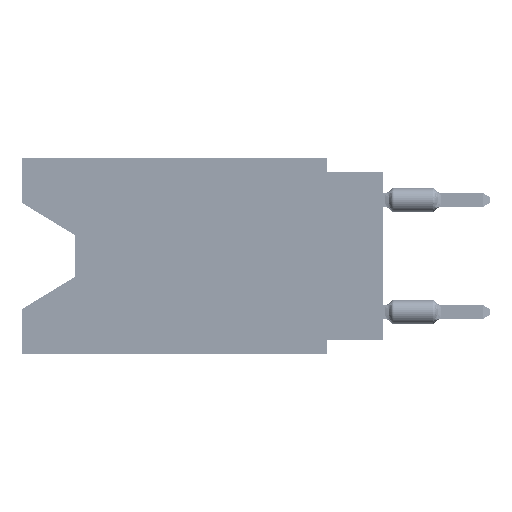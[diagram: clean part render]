
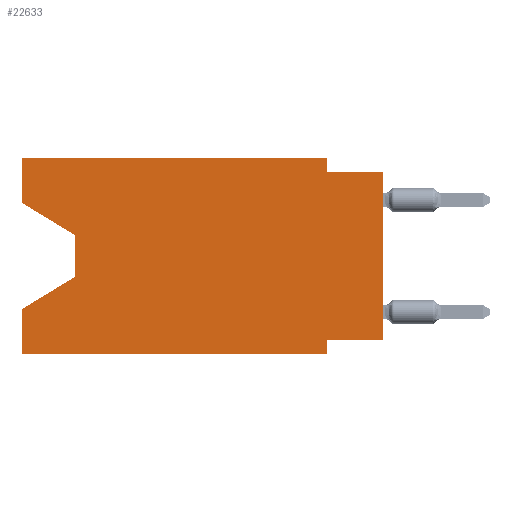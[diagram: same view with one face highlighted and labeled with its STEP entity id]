
A CAD part, left-side view. The second image highlights one B-rep face of the part: STEP entity #22633.
In plain terms, the highlighted planar face has unit normal (-1, 0, 0).
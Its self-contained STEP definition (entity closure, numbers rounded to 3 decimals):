
#1457 = LINE ( 'NONE', #22696, #9150 ) ;
#1768 = VERTEX_POINT ( 'NONE', #43482 ) ;
#1957 = VECTOR ( 'NONE', #57188, 1000. ) ;
#2181 = LINE ( 'NONE', #44290, #11183 ) ;
#2239 = DIRECTION ( 'NONE',  ( 0., 0., 1. ) ) ;
#2450 = EDGE_CURVE ( 'NONE', #53971, #31366, #9779, .T. ) ;
#2933 = EDGE_CURVE ( 'NONE', #52639, #45383, #1457, .T. ) ;
#3321 = DIRECTION ( 'NONE',  ( 0., 0., -1. ) ) ;
#3591 = LINE ( 'NONE', #34068, #43857 ) ;
#5191 = CARTESIAN_POINT ( 'NONE',  ( 0., 13.97, -3.505 ) ) ;
#8055 = CARTESIAN_POINT ( 'NONE',  ( 0., 16.383, 0. ) ) ;
#9150 = VECTOR ( 'NONE', #43224, 1000. ) ;
#9559 = VECTOR ( 'NONE', #39302, 1000. ) ;
#9779 = LINE ( 'NONE', #15256, #10186 ) ;
#10186 = VECTOR ( 'NONE', #26220, 1000. ) ;
#10486 = VERTEX_POINT ( 'NONE', #17986 ) ;
#10541 = FACE_OUTER_BOUND ( 'NONE', #41070, .T. ) ;
#11183 = VECTOR ( 'NONE', #33697, 1000. ) ;
#12348 = DIRECTION ( 'NONE',  ( 0., -1., 0. ) ) ;
#12874 = AXIS2_PLACEMENT_3D ( 'NONE', #35909, #58080, #63221 ) ;
#13448 = EDGE_CURVE ( 'NONE', #23213, #16446, #3591, .T. ) ;
#14159 = LINE ( 'NONE', #40508, #60738 ) ;
#15256 = CARTESIAN_POINT ( 'NONE',  ( 0., 0., -8.255 ) ) ;
#16075 = CARTESIAN_POINT ( 'NONE',  ( 0., 2.54, -8.255 ) ) ;
#16446 = VERTEX_POINT ( 'NONE', #31584 ) ;
#17041 = EDGE_CURVE ( 'NONE', #31366, #42974, #55352, .T. ) ;
#17986 = CARTESIAN_POINT ( 'NONE',  ( 0., 13.97, -3.505 ) ) ;
#18175 = CARTESIAN_POINT ( 'NONE',  ( 0., 16.383, -8.89 ) ) ;
#20119 = EDGE_CURVE ( 'NONE', #1768, #33820, #14159, .T. ) ;
#20193 = CARTESIAN_POINT ( 'NONE',  ( 0., 0., 0. ) ) ;
#20783 = CARTESIAN_POINT ( 'NONE',  ( 0., 2.54, -8.89 ) ) ;
#20844 = CARTESIAN_POINT ( 'NONE',  ( 0., 2.54, 0. ) ) ;
#20927 = VECTOR ( 'NONE', #12348, 1000. ) ;
#22633 = ADVANCED_FACE ( 'NONE', ( #10541 ), #31445, .F. ) ;
#22696 = CARTESIAN_POINT ( 'NONE',  ( 0., 16.383, 0. ) ) ;
#23194 = VECTOR ( 'NONE', #61239, 1000. ) ;
#23213 = VERTEX_POINT ( 'NONE', #60718 ) ;
#26065 = CARTESIAN_POINT ( 'NONE',  ( 0., 0., -0.635 ) ) ;
#26220 = DIRECTION ( 'NONE',  ( 0., 1., 0. ) ) ;
#26972 = CARTESIAN_POINT ( 'NONE',  ( 0., 16.383, 0. ) ) ;
#28565 = ORIENTED_EDGE ( 'NONE', *, *, #2450, .F. ) ;
#31091 = ORIENTED_EDGE ( 'NONE', *, *, #50137, .T. ) ;
#31366 = VERTEX_POINT ( 'NONE', #16075 ) ;
#31445 = PLANE ( 'NONE',  #12874 ) ;
#31584 = CARTESIAN_POINT ( 'NONE',  ( 0., 16.383, -6.852 ) ) ;
#31736 = CARTESIAN_POINT ( 'NONE',  ( 0., 2.54, 0. ) ) ;
#31999 = ORIENTED_EDGE ( 'NONE', *, *, #2933, .F. ) ;
#33697 = DIRECTION ( 'NONE',  ( 0., -0.855, -0.519 ) ) ;
#33820 = VERTEX_POINT ( 'NONE', #26065 ) ;
#33824 = CARTESIAN_POINT ( 'NONE',  ( 0., 2.54, -8.89 ) ) ;
#33839 = CARTESIAN_POINT ( 'NONE',  ( 0., 16.383, 0. ) ) ;
#34068 = CARTESIAN_POINT ( 'NONE',  ( 0., 13.97, -5.385 ) ) ;
#35244 = LINE ( 'NONE', #20844, #57721 ) ;
#35268 = ORIENTED_EDGE ( 'NONE', *, *, #37673, .F. ) ;
#35909 = CARTESIAN_POINT ( 'NONE',  ( 0., 16.383, 0. ) ) ;
#36280 = EDGE_CURVE ( 'NONE', #10486, #23213, #61992, .T. ) ;
#36671 = EDGE_CURVE ( 'NONE', #44117, #1768, #35244, .T. ) ;
#37070 = CARTESIAN_POINT ( 'NONE',  ( 0., 0., -8.255 ) ) ;
#37673 = EDGE_CURVE ( 'NONE', #45383, #44117, #63678, .T. ) ;
#39302 = DIRECTION ( 'NONE',  ( 0., -1., 0. ) ) ;
#40508 = CARTESIAN_POINT ( 'NONE',  ( 0., 0., -0.635 ) ) ;
#41070 = EDGE_LOOP ( 'NONE', ( #53090, #60513, #53792, #55802, #62577, #66275, #28565, #31091, #55437, #60100, #35268, #31999 ) ) ;
#42760 = VECTOR ( 'NONE', #2239, 1000. ) ;
#42974 = VERTEX_POINT ( 'NONE', #20783 ) ;
#43224 = DIRECTION ( 'NONE',  ( 0., 0., 1. ) ) ;
#43482 = CARTESIAN_POINT ( 'NONE',  ( 0., 2.54, -0.635 ) ) ;
#43857 = VECTOR ( 'NONE', #60406, 1000. ) ;
#44117 = VERTEX_POINT ( 'NONE', #31736 ) ;
#44290 = CARTESIAN_POINT ( 'NONE',  ( 0., 16.383, -2.038 ) ) ;
#44846 = LINE ( 'NONE', #20193, #23194 ) ;
#45383 = VERTEX_POINT ( 'NONE', #26972 ) ;
#49137 = LINE ( 'NONE', #8055, #42760 ) ;
#49919 = EDGE_CURVE ( 'NONE', #53029, #42974, #56932, .T. ) ;
#50137 = EDGE_CURVE ( 'NONE', #53971, #33820, #44846, .T. ) ;
#52412 = EDGE_CURVE ( 'NONE', #52639, #10486, #2181, .T. ) ;
#52639 = VERTEX_POINT ( 'NONE', #56217 ) ;
#53029 = VERTEX_POINT ( 'NONE', #62245 ) ;
#53090 = ORIENTED_EDGE ( 'NONE', *, *, #52412, .T. ) ;
#53792 = ORIENTED_EDGE ( 'NONE', *, *, #13448, .T. ) ;
#53971 = VERTEX_POINT ( 'NONE', #37070 ) ;
#55352 = LINE ( 'NONE', #33824, #63717 ) ;
#55437 = ORIENTED_EDGE ( 'NONE', *, *, #20119, .F. ) ;
#55802 = ORIENTED_EDGE ( 'NONE', *, *, #63102, .F. ) ;
#56104 = DIRECTION ( 'NONE',  ( 0., 0., -1. ) ) ;
#56217 = CARTESIAN_POINT ( 'NONE',  ( 0., 16.383, -2.038 ) ) ;
#56932 = LINE ( 'NONE', #18175, #20927 ) ;
#57188 = DIRECTION ( 'NONE',  ( 0., 0., -1. ) ) ;
#57721 = VECTOR ( 'NONE', #56104, 1000. ) ;
#58080 = DIRECTION ( 'NONE',  ( 1., 0., 0. ) ) ;
#60100 = ORIENTED_EDGE ( 'NONE', *, *, #36671, .F. ) ;
#60406 = DIRECTION ( 'NONE',  ( 0., 0.855, -0.519 ) ) ;
#60513 = ORIENTED_EDGE ( 'NONE', *, *, #36280, .T. ) ;
#60718 = CARTESIAN_POINT ( 'NONE',  ( 0., 13.97, -5.385 ) ) ;
#60738 = VECTOR ( 'NONE', #61367, 1000. ) ;
#61239 = DIRECTION ( 'NONE',  ( 0., 0., 1. ) ) ;
#61367 = DIRECTION ( 'NONE',  ( 0., -1., 0. ) ) ;
#61992 = LINE ( 'NONE', #5191, #1957 ) ;
#62245 = CARTESIAN_POINT ( 'NONE',  ( 0., 16.383, -8.89 ) ) ;
#62577 = ORIENTED_EDGE ( 'NONE', *, *, #49919, .T. ) ;
#63102 = EDGE_CURVE ( 'NONE', #53029, #16446, #49137, .T. ) ;
#63221 = DIRECTION ( 'NONE',  ( 0., 0., -1. ) ) ;
#63678 = LINE ( 'NONE', #33839, #9559 ) ;
#63717 = VECTOR ( 'NONE', #3321, 1000. ) ;
#66275 = ORIENTED_EDGE ( 'NONE', *, *, #17041, .F. ) ;
